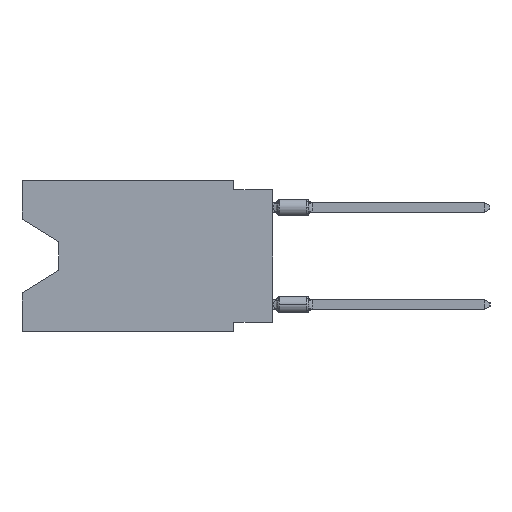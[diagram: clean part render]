
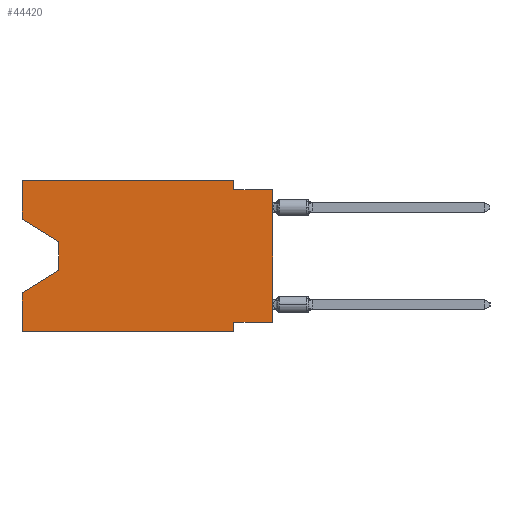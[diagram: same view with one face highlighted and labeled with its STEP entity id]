
A CAD part, left-side view. The second image highlights one B-rep face of the part: STEP entity #44420.
In plain terms, the highlighted planar face has unit normal (-1, 0, 0).
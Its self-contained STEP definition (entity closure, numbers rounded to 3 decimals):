
#577 = VERTEX_POINT ( 'NONE', #5942 ) ;
#739 = LINE ( 'NONE', #26269, #27209 ) ;
#1246 = DIRECTION ( 'NONE',  ( 0., 0.855, -0.519 ) ) ;
#1599 = VECTOR ( 'NONE', #21379, 1000. ) ;
#2154 = VECTOR ( 'NONE', #40685, 1000. ) ;
#3063 = EDGE_CURVE ( 'NONE', #34620, #19461, #45812, .T. ) ;
#3301 = LINE ( 'NONE', #18119, #2154 ) ;
#3987 = EDGE_CURVE ( 'NONE', #18325, #19461, #19713, .T. ) ;
#4420 = CARTESIAN_POINT ( 'NONE',  ( 0., 16.383, -2.546 ) ) ;
#4606 = ORIENTED_EDGE ( 'NONE', *, *, #29570, .T. ) ;
#4662 = LINE ( 'NONE', #4420, #16015 ) ;
#5379 = ORIENTED_EDGE ( 'NONE', *, *, #45784, .F. ) ;
#5942 = CARTESIAN_POINT ( 'NONE',  ( 0., 2.54, -9.271 ) ) ;
#5973 = CARTESIAN_POINT ( 'NONE',  ( 0., 16.383, 0. ) ) ;
#6360 = PLANE ( 'NONE',  #45890 ) ;
#6485 = LINE ( 'NONE', #16458, #27355 ) ;
#6975 = CARTESIAN_POINT ( 'NONE',  ( 0., 0., -0.635 ) ) ;
#9328 = CARTESIAN_POINT ( 'NONE',  ( 0., 13.97, -5.893 ) ) ;
#9339 = CARTESIAN_POINT ( 'NONE',  ( 0., 0., -0.635 ) ) ;
#9586 = CARTESIAN_POINT ( 'NONE',  ( 0., 16.383, -9.906 ) ) ;
#10410 = EDGE_CURVE ( 'NONE', #28296, #40300, #4662, .T. ) ;
#11130 = ORIENTED_EDGE ( 'NONE', *, *, #47949, .F. ) ;
#11374 = VECTOR ( 'NONE', #15474, 1000. ) ;
#11480 = LINE ( 'NONE', #14886, #37264 ) ;
#11828 = LINE ( 'NONE', #26397, #1599 ) ;
#13314 = EDGE_CURVE ( 'NONE', #22031, #40142, #11828, .T. ) ;
#14372 = DIRECTION ( 'NONE',  ( 0., 0., -1. ) ) ;
#14886 = CARTESIAN_POINT ( 'NONE',  ( 0., 16.383, -9.906 ) ) ;
#15128 = DIRECTION ( 'NONE',  ( 0., -0.855, -0.519 ) ) ;
#15474 = DIRECTION ( 'NONE',  ( 0., 0., -1. ) ) ;
#15744 = VECTOR ( 'NONE', #35605, 1000. ) ;
#15806 = DIRECTION ( 'NONE',  ( 0., 1., 0. ) ) ;
#16015 = VECTOR ( 'NONE', #15128, 1000. ) ;
#16458 = CARTESIAN_POINT ( 'NONE',  ( 0., 2.54, -9.906 ) ) ;
#18119 = CARTESIAN_POINT ( 'NONE',  ( 0., 16.383, 0. ) ) ;
#18325 = VERTEX_POINT ( 'NONE', #9328 ) ;
#18962 = EDGE_CURVE ( 'NONE', #30602, #25991, #36699, .T. ) ;
#19461 = VERTEX_POINT ( 'NONE', #27090 ) ;
#19584 = CARTESIAN_POINT ( 'NONE',  ( 0., 13.97, -4.013 ) ) ;
#19590 = ORIENTED_EDGE ( 'NONE', *, *, #41646, .T. ) ;
#19713 = LINE ( 'NONE', #34541, #22791 ) ;
#20749 = LINE ( 'NONE', #9339, #34078 ) ;
#21379 = DIRECTION ( 'NONE',  ( 0., 0., 1. ) ) ;
#21797 = ORIENTED_EDGE ( 'NONE', *, *, #3987, .T. ) ;
#22031 = VERTEX_POINT ( 'NONE', #33032 ) ;
#22143 = DIRECTION ( 'NONE',  ( 1., 0., 0. ) ) ;
#22409 = DIRECTION ( 'NONE',  ( 0., -1., 0. ) ) ;
#22519 = ORIENTED_EDGE ( 'NONE', *, *, #32658, .F. ) ;
#22791 = VECTOR ( 'NONE', #1246, 1000. ) ;
#23104 = DIRECTION ( 'NONE',  ( 0., -1., 0. ) ) ;
#25803 = LINE ( 'NONE', #40596, #33690 ) ;
#25991 = VERTEX_POINT ( 'NONE', #30990 ) ;
#26269 = CARTESIAN_POINT ( 'NONE',  ( 0., 0., -9.271 ) ) ;
#26397 = CARTESIAN_POINT ( 'NONE',  ( 0., 0., 0. ) ) ;
#27090 = CARTESIAN_POINT ( 'NONE',  ( 0., 16.383, -7.36 ) ) ;
#27209 = VECTOR ( 'NONE', #15806, 1000. ) ;
#27355 = VECTOR ( 'NONE', #46082, 1000. ) ;
#28136 = CARTESIAN_POINT ( 'NONE',  ( 0., 2.54, 0. ) ) ;
#28274 = DIRECTION ( 'NONE',  ( 0., -1., 0. ) ) ;
#28296 = VERTEX_POINT ( 'NONE', #35720 ) ;
#28458 = FACE_OUTER_BOUND ( 'NONE', #29694, .T. ) ;
#29570 = EDGE_CURVE ( 'NONE', #40300, #18325, #41452, .T. ) ;
#29694 = EDGE_LOOP ( 'NONE', ( #42282, #4606, #21797, #33320, #19590, #5379, #30568, #39415, #22519, #35882, #11130, #37341 ) ) ;
#30568 = ORIENTED_EDGE ( 'NONE', *, *, #36603, .F. ) ;
#30602 = VERTEX_POINT ( 'NONE', #28136 ) ;
#30756 = CARTESIAN_POINT ( 'NONE',  ( 0., 13.97, -4.013 ) ) ;
#30990 = CARTESIAN_POINT ( 'NONE',  ( 0., 2.54, -0.635 ) ) ;
#31096 = EDGE_CURVE ( 'NONE', #28296, #37849, #3301, .T. ) ;
#32658 = EDGE_CURVE ( 'NONE', #25991, #40142, #20749, .T. ) ;
#33032 = CARTESIAN_POINT ( 'NONE',  ( 0., 0., -9.271 ) ) ;
#33320 = ORIENTED_EDGE ( 'NONE', *, *, #3063, .F. ) ;
#33650 = VECTOR ( 'NONE', #14372, 1000. ) ;
#33690 = VECTOR ( 'NONE', #23104, 1000. ) ;
#34078 = VECTOR ( 'NONE', #28274, 1000. ) ;
#34541 = CARTESIAN_POINT ( 'NONE',  ( 0., 13.97, -5.893 ) ) ;
#34620 = VERTEX_POINT ( 'NONE', #9586 ) ;
#35605 = DIRECTION ( 'NONE',  ( 0., 0., 1. ) ) ;
#35720 = CARTESIAN_POINT ( 'NONE',  ( 0., 16.383, -2.546 ) ) ;
#35882 = ORIENTED_EDGE ( 'NONE', *, *, #18962, .F. ) ;
#35980 = CARTESIAN_POINT ( 'NONE',  ( 0., 2.54, -9.906 ) ) ;
#36603 = EDGE_CURVE ( 'NONE', #22031, #577, #739, .T. ) ;
#36699 = LINE ( 'NONE', #43496, #33650 ) ;
#37264 = VECTOR ( 'NONE', #22409, 1000. ) ;
#37341 = ORIENTED_EDGE ( 'NONE', *, *, #31096, .F. ) ;
#37849 = VERTEX_POINT ( 'NONE', #40112 ) ;
#39415 = ORIENTED_EDGE ( 'NONE', *, *, #13314, .T. ) ;
#40112 = CARTESIAN_POINT ( 'NONE',  ( 0., 16.383, 0. ) ) ;
#40142 = VERTEX_POINT ( 'NONE', #6975 ) ;
#40300 = VERTEX_POINT ( 'NONE', #30756 ) ;
#40578 = DIRECTION ( 'NONE',  ( 0., 0., -1. ) ) ;
#40596 = CARTESIAN_POINT ( 'NONE',  ( 0., 16.383, 0. ) ) ;
#40685 = DIRECTION ( 'NONE',  ( 0., 0., 1. ) ) ;
#41452 = LINE ( 'NONE', #19584, #11374 ) ;
#41646 = EDGE_CURVE ( 'NONE', #34620, #43076, #11480, .T. ) ;
#42282 = ORIENTED_EDGE ( 'NONE', *, *, #10410, .T. ) ;
#43076 = VERTEX_POINT ( 'NONE', #35980 ) ;
#43496 = CARTESIAN_POINT ( 'NONE',  ( 0., 2.54, 0. ) ) ;
#44420 = ADVANCED_FACE ( 'NONE', ( #28458 ), #6360, .F. ) ;
#45415 = CARTESIAN_POINT ( 'NONE',  ( 0., 16.383, 0. ) ) ;
#45784 = EDGE_CURVE ( 'NONE', #577, #43076, #6485, .T. ) ;
#45812 = LINE ( 'NONE', #5973, #15744 ) ;
#45890 = AXIS2_PLACEMENT_3D ( 'NONE', #45415, #22143, #40578 ) ;
#46082 = DIRECTION ( 'NONE',  ( 0., 0., -1. ) ) ;
#47949 = EDGE_CURVE ( 'NONE', #37849, #30602, #25803, .T. ) ;
